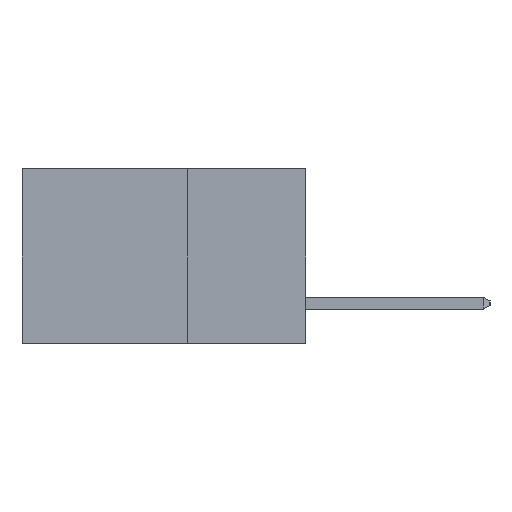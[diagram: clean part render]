
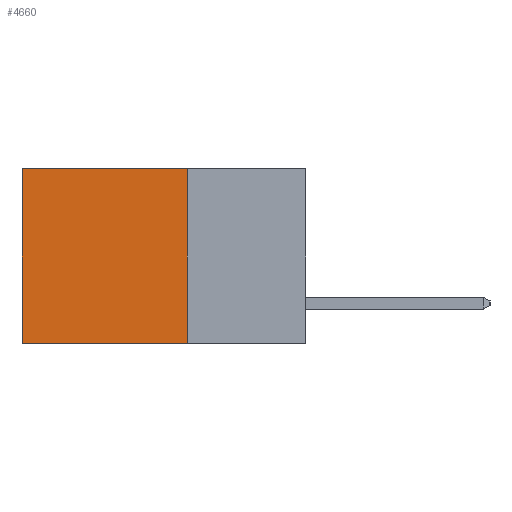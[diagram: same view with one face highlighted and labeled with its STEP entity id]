
A CAD part, left-side view. The second image highlights one B-rep face of the part: STEP entity #4660.
In plain terms, the highlighted planar face has unit normal (-1, 0, 0).
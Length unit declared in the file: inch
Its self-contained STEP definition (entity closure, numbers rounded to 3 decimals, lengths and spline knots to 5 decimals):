
#533 = ORIENTED_EDGE ( 'NONE', *, *, #811, .T. ) ;
#811 = EDGE_CURVE ( 'NONE', #5565, #988, #8626, .T. ) ;
#984 = DIRECTION ( 'NONE',  ( 0., 0., -1. ) ) ;
#988 = VERTEX_POINT ( 'NONE', #1249 ) ;
#1002 = DIRECTION ( 'NONE',  ( 1., 0., 0. ) ) ;
#1072 = CARTESIAN_POINT ( 'NONE',  ( 0.2615, 0.25, -0.37 ) ) ;
#1120 = VERTEX_POINT ( 'NONE', #7039 ) ;
#1216 = DIRECTION ( 'NONE',  ( 0., 0., -1. ) ) ;
#1249 = CARTESIAN_POINT ( 'NONE',  ( 0.2615, 0.6, -0.37 ) ) ;
#1664 = PLANE ( 'NONE',  #3403 ) ;
#1997 = EDGE_CURVE ( 'NONE', #3230, #1120, #8605, .T. ) ;
#2169 = CARTESIAN_POINT ( 'NONE',  ( 0.2615, 0.6, 0. ) ) ;
#2647 = EDGE_LOOP ( 'NONE', ( #533, #3030, #3730, #4827 ) ) ;
#3030 = ORIENTED_EDGE ( 'NONE', *, *, #5077, .F. ) ;
#3230 = VERTEX_POINT ( 'NONE', #8685 ) ;
#3403 = AXIS2_PLACEMENT_3D ( 'NONE', #1072, #1002, #984 ) ;
#3730 = ORIENTED_EDGE ( 'NONE', *, *, #1997, .F. ) ;
#4481 = LINE ( 'NONE', #7781, #6314 ) ;
#4660 = ADVANCED_FACE ( 'NONE', ( #5886 ), #1664, .F. ) ;
#4827 = ORIENTED_EDGE ( 'NONE', *, *, #7625, .T. ) ;
#4979 = VECTOR ( 'NONE', #5600, 39.37008 ) ;
#5073 = VECTOR ( 'NONE', #8462, 39.37008 ) ;
#5077 = EDGE_CURVE ( 'NONE', #1120, #988, #4481, .T. ) ;
#5191 = LINE ( 'NONE', #5635, #4979 ) ;
#5565 = VERTEX_POINT ( 'NONE', #2169 ) ;
#5600 = DIRECTION ( 'NONE',  ( 0., 1., 0. ) ) ;
#5635 = CARTESIAN_POINT ( 'NONE',  ( 0.2615, 0.25, 0. ) ) ;
#5886 = FACE_OUTER_BOUND ( 'NONE', #2647, .T. ) ;
#6314 = VECTOR ( 'NONE', #7525, 39.37008 ) ;
#6984 = CARTESIAN_POINT ( 'NONE',  ( 0.2615, 0.25, -0.37 ) ) ;
#7039 = CARTESIAN_POINT ( 'NONE',  ( 0.2615, 0.25, -0.37 ) ) ;
#7299 = VECTOR ( 'NONE', #1216, 39.37008 ) ;
#7525 = DIRECTION ( 'NONE',  ( 0., 1., 0. ) ) ;
#7625 = EDGE_CURVE ( 'NONE', #3230, #5565, #5191, .T. ) ;
#7781 = CARTESIAN_POINT ( 'NONE',  ( 0.2615, 0.25, -0.37 ) ) ;
#7837 = CARTESIAN_POINT ( 'NONE',  ( 0.2615, 0.6, -0.37 ) ) ;
#8462 = DIRECTION ( 'NONE',  ( 0., 0., -1. ) ) ;
#8605 = LINE ( 'NONE', #6984, #7299 ) ;
#8626 = LINE ( 'NONE', #7837, #5073 ) ;
#8685 = CARTESIAN_POINT ( 'NONE',  ( 0.2615, 0.25, 0. ) ) ;
